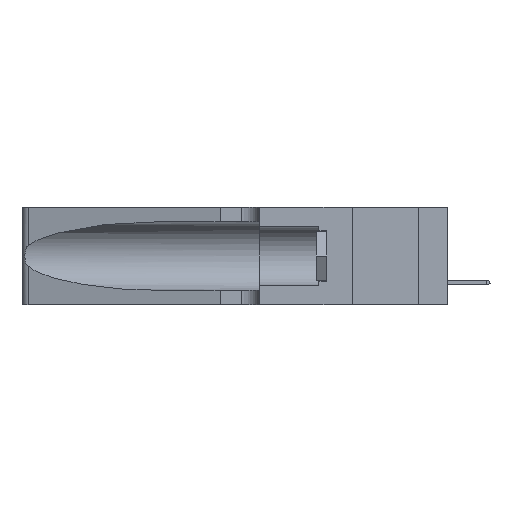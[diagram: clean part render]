
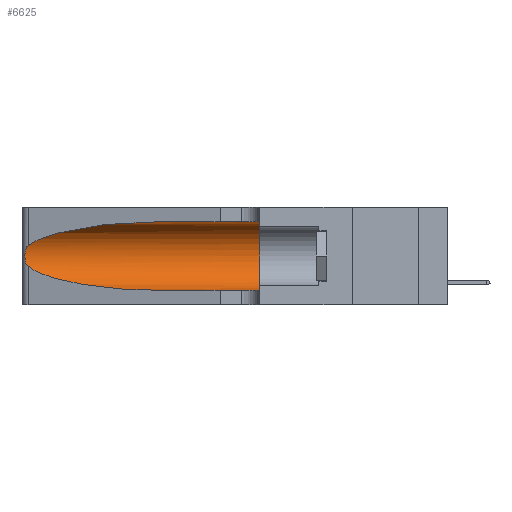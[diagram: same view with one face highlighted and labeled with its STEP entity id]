
A CAD part, left-side view. The second image highlights one B-rep face of the part: STEP entity #6625.
In plain terms, the highlighted cylindrical face has radius 3.308 mm (diameter 6.617 mm), a partial arc.
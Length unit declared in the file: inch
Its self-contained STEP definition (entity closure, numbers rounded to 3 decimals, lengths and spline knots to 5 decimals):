
#308 = CARTESIAN_POINT ( 'NONE',  ( 0.1305, 0.72297, 0.05475 ) ) ;
#952 = CARTESIAN_POINT ( 'NONE',  ( 0.26075, 1.23896, 0.178 ) ) ;
#1134 = VERTEX_POINT ( 'NONE', #308 ) ;
#1159 = CARTESIAN_POINT ( 'NONE',  ( 0.25487, 1.22718, 0.22369 ) ) ;
#1276 = EDGE_CURVE ( 'NONE', #1134, #18254, #2111, .T. ) ;
#1324 = VERTEX_POINT ( 'NONE', #9376 ) ;
#1468 = ORIENTED_EDGE ( 'NONE', *, *, #14667, .T. ) ;
#1641 = CARTESIAN_POINT ( 'NONE',  ( 0.18966, 0.96281, 0.31525 ) ) ;
#1949 = EDGE_CURVE ( 'NONE', #1324, #1134, #20340, .T. ) ;
#2111 = LINE ( 'NONE', #12830, #8704 ) ;
#2492 = EDGE_LOOP ( 'NONE', ( #1468, #12583, #3241, #4298, #9473, #18651 ) ) ;
#2577 = CARTESIAN_POINT ( 'NONE',  ( 0.25856, 1.23593, 0.16098 ) ) ;
#2789 = CARTESIAN_POINT ( 'NONE',  ( 0.26075, 1.23896, 0.19203 ) ) ;
#3241 = ORIENTED_EDGE ( 'NONE', *, *, #1949, .T. ) ;
#3648 = AXIS2_PLACEMENT_3D ( 'NONE', #17353, #15649, #20436 ) ;
#3816 = LINE ( 'NONE', #14522, #16225 ) ;
#4298 = ORIENTED_EDGE ( 'NONE', *, *, #1276, .T. ) ;
#4882 = CARTESIAN_POINT ( 'NONE',  ( 0.18966, 0.96281, 0.05475 ) ) ;
#5814 = DIRECTION ( 'NONE',  ( 0., 1., 0. ) ) ;
#5983 = VERTEX_POINT ( 'NONE', #9343 ) ;
#6064 = EDGE_CURVE ( 'NONE', #8089, #18254, #14115, .T. ) ;
#6357 = CARTESIAN_POINT ( 'NONE',  ( 0.25487, 1.22718, 0.22369 ) ) ;
#6472 = CARTESIAN_POINT ( 'NONE',  ( 0.1305, 0.72297, 0.05475 ) ) ;
#6625 = ADVANCED_FACE ( 'NONE', ( #18146 ), #10547, .F. ) ;
#7385 = CARTESIAN_POINT ( 'NONE',  ( 0.25555, 1.22994, 0.2215 ) ) ;
#7592 = CARTESIAN_POINT ( 'NONE',  ( 0.25639, 1.23184, 0.21858 ) ) ;
#7652 = CARTESIAN_POINT ( 'NONE',  ( 0.25487, 1.22718, 0.22369 ) ) ;
#8089 = VERTEX_POINT ( 'NONE', #13081 ) ;
#8509 = VERTEX_POINT ( 'NONE', #7652 ) ;
#8704 = VECTOR ( 'NONE', #14275, 39.37008 ) ;
#9130 = CARTESIAN_POINT ( 'NONE',  ( 0.1305, 0.35, 0.185 ) ) ;
#9289 = CARTESIAN_POINT ( 'NONE',  ( 0.25789, 1.23486, 0.15765 ) ) ;
#9343 = CARTESIAN_POINT ( 'NONE',  ( 0.1305, 0.72297, 0.31525 ) ) ;
#9376 = CARTESIAN_POINT ( 'NONE',  ( 0.25487, 1.22718, 0.14631 ) ) ;
#9473 = ORIENTED_EDGE ( 'NONE', *, *, #6064, .F. ) ;
#9654 = CARTESIAN_POINT ( 'NONE',  ( 0.1305, 0.72297, 0.31525 ) ) ;
#9973 = B_SPLINE_CURVE_WITH_KNOTS ( 'NONE', 3,
 ( #1159, #7385, #7592, #12498, #18727, #10663, #2789, #952, #19011, #2577, #9289, #12217, #13902, #17143 ),
 .UNSPECIFIED., .F., .F.,
 ( 4, 2, 2, 2, 2, 2, 4 ),
 ( 0., 0.00027, 0.00053, 0.00107, 0.0016, 0.00187, 0.00214 ),
 .UNSPECIFIED. ) ;
#10547 = CYLINDRICAL_SURFACE ( 'NONE', #3648, 0.13025 ) ;
#10663 = CARTESIAN_POINT ( 'NONE',  ( 0.26018, 1.23835, 0.19895 ) ) ;
#11463 = CARTESIAN_POINT ( 'NONE',  ( 0.2373, 1.15595, 0.08982 ) ) ;
#11936 = AXIS2_PLACEMENT_3D ( 'NONE', #9130, #5814, #20363 ) ;
#11970 = EDGE_CURVE ( 'NONE', #5983, #8089, #3816, .T. ) ;
#12217 = CARTESIAN_POINT ( 'NONE',  ( 0.25639, 1.23186, 0.15144 ) ) ;
#12498 = CARTESIAN_POINT ( 'NONE',  ( 0.25787, 1.23484, 0.2124 ) ) ;
#12583 = ORIENTED_EDGE ( 'NONE', *, *, #15546, .T. ) ;
#12830 = CARTESIAN_POINT ( 'NONE',  ( 0.1305, 1.61858, 0.05475 ) ) ;
#13081 = CARTESIAN_POINT ( 'NONE',  ( 0.1305, 0.35, 0.31525 ) ) ;
#13902 = CARTESIAN_POINT ( 'NONE',  ( 0.25555, 1.22993, 0.14849 ) ) ;
#14115 = CIRCLE ( 'NONE', #11936, 0.13025 ) ;
#14275 = DIRECTION ( 'NONE',  ( 0., -1., 0. ) ) ;
#14522 = CARTESIAN_POINT ( 'NONE',  ( 0.1305, 1.61858, 0.31525 ) ) ;
#14667 = EDGE_CURVE ( 'NONE', #5983, #8509, #15275, .T. ) ;
#15275 =( BOUNDED_CURVE ( )  B_SPLINE_CURVE ( 3, ( #9654, #1641, #15938, #6357 ),
 .UNSPECIFIED., .F., .F. ) 
 B_SPLINE_CURVE_WITH_KNOTS ( ( 4, 4 ),
 ( 1.5708, 2.84003 ),
 .UNSPECIFIED. ) 
 CURVE ( )  GEOMETRIC_REPRESENTATION_ITEM ( )  RATIONAL_B_SPLINE_CURVE ( ( 1., 0.87, 0.87, 1. ) ) 
 REPRESENTATION_ITEM ( '' )  );
#15546 = EDGE_CURVE ( 'NONE', #8509, #1324, #9973, .T. ) ;
#15649 = DIRECTION ( 'NONE',  ( 0., -1., 0. ) ) ;
#15938 = CARTESIAN_POINT ( 'NONE',  ( 0.2373, 1.15595, 0.28018 ) ) ;
#16225 = VECTOR ( 'NONE', #19483, 39.37008 ) ;
#16388 = CARTESIAN_POINT ( 'NONE',  ( 0.25487, 1.22718, 0.14631 ) ) ;
#17143 = CARTESIAN_POINT ( 'NONE',  ( 0.25487, 1.22718, 0.14631 ) ) ;
#17353 = CARTESIAN_POINT ( 'NONE',  ( 0.1305, 1.61858, 0.185 ) ) ;
#18146 = FACE_OUTER_BOUND ( 'NONE', #2492, .T. ) ;
#18172 = CARTESIAN_POINT ( 'NONE',  ( 0.1305, 0.35, 0.05475 ) ) ;
#18254 = VERTEX_POINT ( 'NONE', #18172 ) ;
#18651 = ORIENTED_EDGE ( 'NONE', *, *, #11970, .F. ) ;
#18727 = CARTESIAN_POINT ( 'NONE',  ( 0.25854, 1.2359, 0.20912 ) ) ;
#19011 = CARTESIAN_POINT ( 'NONE',  ( 0.26017, 1.23833, 0.17102 ) ) ;
#19483 = DIRECTION ( 'NONE',  ( 0., -1., 0. ) ) ;
#20340 =( BOUNDED_CURVE ( )  B_SPLINE_CURVE ( 3, ( #16388, #11463, #4882, #6472 ),
 .UNSPECIFIED., .F., .T. ) 
 B_SPLINE_CURVE_WITH_KNOTS ( ( 4, 4 ),
 ( 3.44316, 4.71239 ),
 .UNSPECIFIED. ) 
 CURVE ( )  GEOMETRIC_REPRESENTATION_ITEM ( )  RATIONAL_B_SPLINE_CURVE ( ( 1., 0.87, 0.87, 1. ) ) 
 REPRESENTATION_ITEM ( '' )  );
#20363 = DIRECTION ( 'NONE',  ( 0., 0., 1. ) ) ;
#20436 = DIRECTION ( 'NONE',  ( 0., 0., -1. ) ) ;
